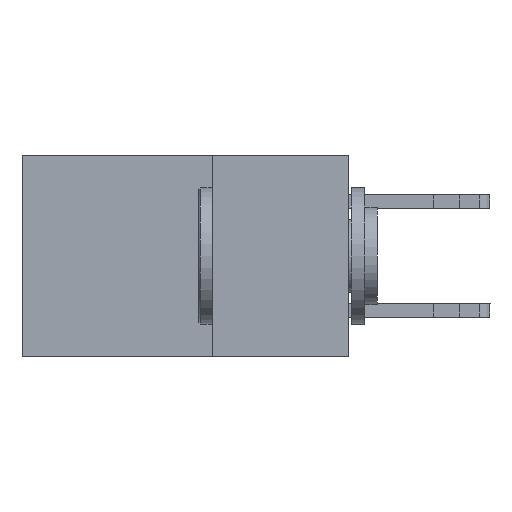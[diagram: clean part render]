
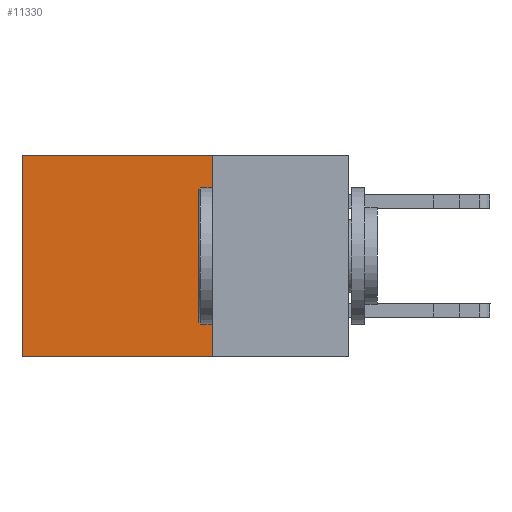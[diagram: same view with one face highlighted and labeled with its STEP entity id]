
A CAD part, left-side view. The second image highlights one B-rep face of the part: STEP entity #11330.
In plain terms, the highlighted planar face has unit normal (-1, 0, 0).
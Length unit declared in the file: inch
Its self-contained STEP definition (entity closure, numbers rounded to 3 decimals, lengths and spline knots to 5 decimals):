
#169 = LINE ( 'NONE', #1789, #11587 ) ;
#725 = AXIS2_PLACEMENT_3D ( 'NONE', #22611, #10021, #9917 ) ;
#852 = FACE_OUTER_BOUND ( 'NONE', #8265, .T. ) ;
#1789 = CARTESIAN_POINT ( 'NONE',  ( 0.298, 0.25, 0. ) ) ;
#3208 = CARTESIAN_POINT ( 'NONE',  ( 0.298, 0.25, 0. ) ) ;
#3750 = EDGE_CURVE ( 'NONE', #13975, #19982, #6434, .T. ) ;
#6434 = LINE ( 'NONE', #14890, #24698 ) ;
#6703 = CARTESIAN_POINT ( 'NONE',  ( 0.298, 0.6, 0. ) ) ;
#8169 = ORIENTED_EDGE ( 'NONE', *, *, #3750, .F. ) ;
#8265 = EDGE_LOOP ( 'NONE', ( #21671, #8169, #20673, #8555 ) ) ;
#8555 = ORIENTED_EDGE ( 'NONE', *, *, #15282, .T. ) ;
#8695 = DIRECTION ( 'NONE',  ( 0., 1., 0. ) ) ;
#9917 = DIRECTION ( 'NONE',  ( 0., 0., -1. ) ) ;
#10021 = DIRECTION ( 'NONE',  ( 1., 0., 0. ) ) ;
#10161 = VERTEX_POINT ( 'NONE', #26903 ) ;
#11330 = ADVANCED_FACE ( 'NONE', ( #852 ), #16310, .F. ) ;
#11587 = VECTOR ( 'NONE', #26019, 39.37008 ) ;
#12137 = EDGE_CURVE ( 'NONE', #17029, #13975, #169, .T. ) ;
#12650 = VECTOR ( 'NONE', #18567, 39.37008 ) ;
#13358 = VECTOR ( 'NONE', #26149, 39.37008 ) ;
#13975 = VERTEX_POINT ( 'NONE', #16222 ) ;
#14344 = LINE ( 'NONE', #3208, #12650 ) ;
#14369 = EDGE_CURVE ( 'NONE', #10161, #19982, #20854, .T. ) ;
#14890 = CARTESIAN_POINT ( 'NONE',  ( 0.298, 0.25, -0.37 ) ) ;
#15282 = EDGE_CURVE ( 'NONE', #17029, #10161, #14344, .T. ) ;
#16222 = CARTESIAN_POINT ( 'NONE',  ( 0.298, 0.25, -0.37 ) ) ;
#16310 = PLANE ( 'NONE',  #725 ) ;
#17029 = VERTEX_POINT ( 'NONE', #18792 ) ;
#18567 = DIRECTION ( 'NONE',  ( 0., 1., 0. ) ) ;
#18792 = CARTESIAN_POINT ( 'NONE',  ( 0.298, 0.25, 0. ) ) ;
#19982 = VERTEX_POINT ( 'NONE', #23590 ) ;
#20673 = ORIENTED_EDGE ( 'NONE', *, *, #12137, .F. ) ;
#20854 = LINE ( 'NONE', #6703, #13358 ) ;
#21671 = ORIENTED_EDGE ( 'NONE', *, *, #14369, .T. ) ;
#22611 = CARTESIAN_POINT ( 'NONE',  ( 0.298, 0.25, 0. ) ) ;
#23590 = CARTESIAN_POINT ( 'NONE',  ( 0.298, 0.6, -0.37 ) ) ;
#24698 = VECTOR ( 'NONE', #8695, 39.37008 ) ;
#26019 = DIRECTION ( 'NONE',  ( 0., 0., -1. ) ) ;
#26149 = DIRECTION ( 'NONE',  ( 0., 0., -1. ) ) ;
#26903 = CARTESIAN_POINT ( 'NONE',  ( 0.298, 0.6, 0. ) ) ;
